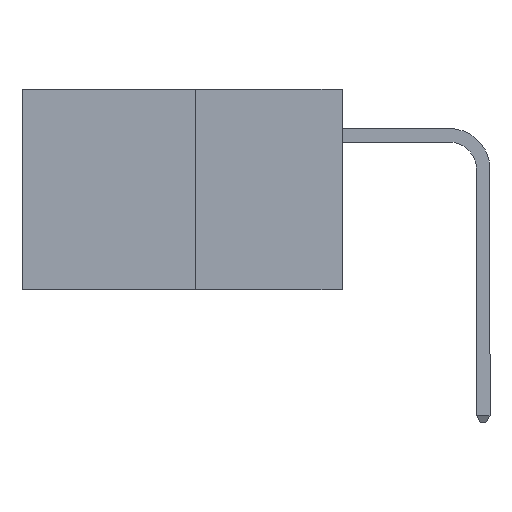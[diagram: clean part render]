
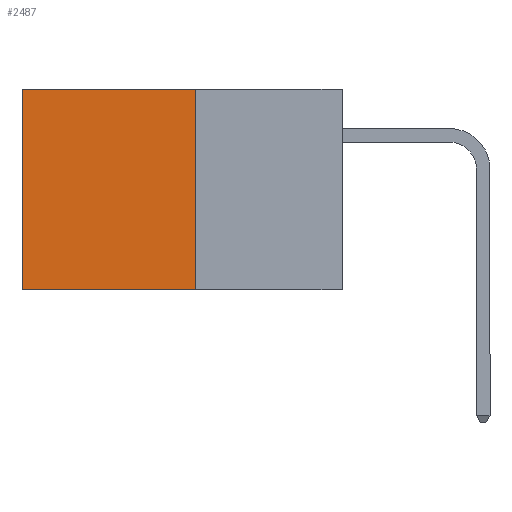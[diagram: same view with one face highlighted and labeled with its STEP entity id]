
A CAD part, left-side view. The second image highlights one B-rep face of the part: STEP entity #2487.
In plain terms, the highlighted planar face has unit normal (-1, 0, 0).
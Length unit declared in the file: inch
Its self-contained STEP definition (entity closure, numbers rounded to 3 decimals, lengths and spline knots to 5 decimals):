
#496 = DIRECTION ( 'NONE',  ( 0., 1., 0. ) ) ;
#534 = CARTESIAN_POINT ( 'NONE',  ( 0.277, 0.27, -0.37 ) ) ;
#558 = CARTESIAN_POINT ( 'NONE',  ( 0.277, 0.27, -0.37 ) ) ;
#1449 = CARTESIAN_POINT ( 'NONE',  ( 0.277, 0.59, -0.37 ) ) ;
#1632 = EDGE_CURVE ( 'NONE', #9418, #7369, #6818, .T. ) ;
#2048 = VECTOR ( 'NONE', #496, 39.37008 ) ;
#2297 = EDGE_LOOP ( 'NONE', ( #8253, #5889, #7500, #5692 ) ) ;
#2487 = ADVANCED_FACE ( 'NONE', ( #10848 ), #7882, .F. ) ;
#3285 = DIRECTION ( 'NONE',  ( 0., 0., -1. ) ) ;
#3808 = CARTESIAN_POINT ( 'NONE',  ( 0.277, 0.27, -0.37 ) ) ;
#4168 = VECTOR ( 'NONE', #7978, 39.37008 ) ;
#4917 = VERTEX_POINT ( 'NONE', #8894 ) ;
#4960 = EDGE_CURVE ( 'NONE', #11804, #7369, #10629, .T. ) ;
#5002 = EDGE_CURVE ( 'NONE', #4917, #9418, #5380, .T. ) ;
#5073 = EDGE_CURVE ( 'NONE', #4917, #11804, #11633, .T. ) ;
#5380 = LINE ( 'NONE', #3808, #10039 ) ;
#5692 = ORIENTED_EDGE ( 'NONE', *, *, #5073, .T. ) ;
#5889 = ORIENTED_EDGE ( 'NONE', *, *, #1632, .F. ) ;
#6106 = CARTESIAN_POINT ( 'NONE',  ( 0.277, 0.59, 0. ) ) ;
#6179 = AXIS2_PLACEMENT_3D ( 'NONE', #8325, #9480, #8714 ) ;
#6818 = LINE ( 'NONE', #534, #2048 ) ;
#7300 = CARTESIAN_POINT ( 'NONE',  ( 0.277, 0.27, 0. ) ) ;
#7369 = VERTEX_POINT ( 'NONE', #11720 ) ;
#7500 = ORIENTED_EDGE ( 'NONE', *, *, #5002, .F. ) ;
#7882 = PLANE ( 'NONE',  #6179 ) ;
#7978 = DIRECTION ( 'NONE',  ( 0., 1., 0. ) ) ;
#8253 = ORIENTED_EDGE ( 'NONE', *, *, #4960, .T. ) ;
#8325 = CARTESIAN_POINT ( 'NONE',  ( 0.277, 0.27, -0.37 ) ) ;
#8590 = DIRECTION ( 'NONE',  ( 0., 0., -1. ) ) ;
#8714 = DIRECTION ( 'NONE',  ( 0., 0., -1. ) ) ;
#8894 = CARTESIAN_POINT ( 'NONE',  ( 0.277, 0.27, 0. ) ) ;
#9418 = VERTEX_POINT ( 'NONE', #558 ) ;
#9480 = DIRECTION ( 'NONE',  ( 1., 0., 0. ) ) ;
#10039 = VECTOR ( 'NONE', #3285, 39.37008 ) ;
#10344 = VECTOR ( 'NONE', #8590, 39.37008 ) ;
#10629 = LINE ( 'NONE', #1449, #10344 ) ;
#10848 = FACE_OUTER_BOUND ( 'NONE', #2297, .T. ) ;
#11633 = LINE ( 'NONE', #7300, #4168 ) ;
#11720 = CARTESIAN_POINT ( 'NONE',  ( 0.277, 0.59, -0.37 ) ) ;
#11804 = VERTEX_POINT ( 'NONE', #6106 ) ;
